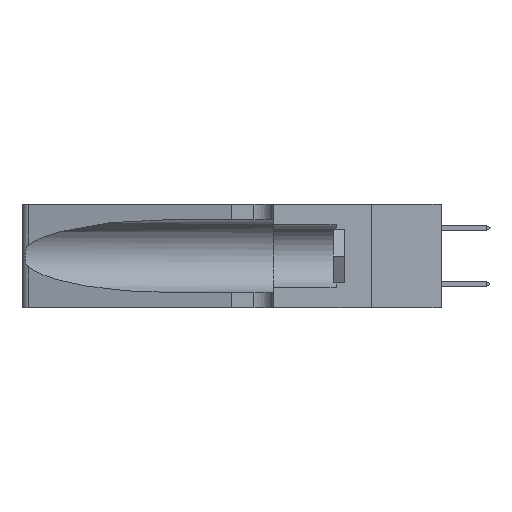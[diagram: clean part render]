
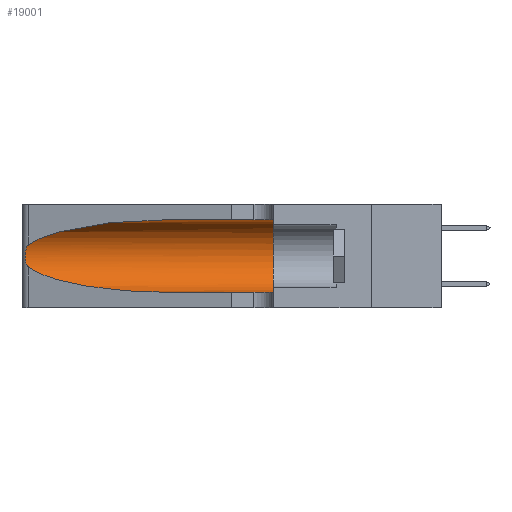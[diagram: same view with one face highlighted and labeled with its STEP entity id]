
A CAD part, left-side view. The second image highlights one B-rep face of the part: STEP entity #19001.
In plain terms, the highlighted cylindrical face has radius 3.308 mm (diameter 6.617 mm), a partial arc.
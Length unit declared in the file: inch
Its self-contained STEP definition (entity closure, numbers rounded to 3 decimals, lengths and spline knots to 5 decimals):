
#551 = ORIENTED_EDGE ( 'NONE', *, *, #17460, .T. ) ;
#641 = CARTESIAN_POINT ( 'NONE',  ( 0.25487, 1.22718, 0.14631 ) ) ;
#1133 =( BOUNDED_CURVE ( )  B_SPLINE_CURVE ( 3, ( #2060, #19327, #19222, #4439 ),
 .UNSPECIFIED., .F., .T. ) 
 B_SPLINE_CURVE_WITH_KNOTS ( ( 4, 4 ),
 ( 1.5708, 2.84003 ),
 .UNSPECIFIED. ) 
 CURVE ( )  GEOMETRIC_REPRESENTATION_ITEM ( )  RATIONAL_B_SPLINE_CURVE ( ( 1., 0.87, 0.87, 1. ) ) 
 REPRESENTATION_ITEM ( '' )  );
#1561 = CARTESIAN_POINT ( 'NONE',  ( 0.25555, 1.22993, 0.14849 ) ) ;
#1677 = CARTESIAN_POINT ( 'NONE',  ( 0.1305, 0.35, 0.185 ) ) ;
#1917 = EDGE_LOOP ( 'NONE', ( #7066, #551, #21271, #15717, #28326, #12097 ) ) ;
#2060 = CARTESIAN_POINT ( 'NONE',  ( 0.1305, 0.72297, 0.31525 ) ) ;
#2667 = EDGE_CURVE ( 'NONE', #29819, #5821, #16450, .T. ) ;
#3539 = FACE_OUTER_BOUND ( 'NONE', #1917, .T. ) ;
#4139 = VERTEX_POINT ( 'NONE', #7620 ) ;
#4439 = CARTESIAN_POINT ( 'NONE',  ( 0.25487, 1.22718, 0.22369 ) ) ;
#4511 = B_SPLINE_CURVE_WITH_KNOTS ( 'NONE', 3,
 ( #25887, #30851, #11072, #16334, #6303, #11182, #23590, #28400, #13532, #23703, #26225, #11397, #1561, #16020 ),
 .UNSPECIFIED., .F., .F.,
 ( 4, 2, 2, 2, 2, 2, 4 ),
 ( 0., 0.00027, 0.00053, 0.00107, 0.0016, 0.00187, 0.00214 ),
 .UNSPECIFIED. ) ;
#4860 = EDGE_CURVE ( 'NONE', #20494, #13696, #8228, .T. ) ;
#4925 = CARTESIAN_POINT ( 'NONE',  ( 0.1305, 0.35, 0.05475 ) ) ;
#5821 = VERTEX_POINT ( 'NONE', #4925 ) ;
#6303 = CARTESIAN_POINT ( 'NONE',  ( 0.25854, 1.2359, 0.20912 ) ) ;
#7066 = ORIENTED_EDGE ( 'NONE', *, *, #11610, .T. ) ;
#7512 = VERTEX_POINT ( 'NONE', #26462 ) ;
#7620 = CARTESIAN_POINT ( 'NONE',  ( 0.25487, 1.22718, 0.22369 ) ) ;
#8002 = CARTESIAN_POINT ( 'NONE',  ( 0.18966, 0.96281, 0.05475 ) ) ;
#8224 = DIRECTION ( 'NONE',  ( 0., -1., 0. ) ) ;
#8228 = LINE ( 'NONE', #12948, #19827 ) ;
#8367 = DIRECTION ( 'NONE',  ( 0., -1., 0. ) ) ;
#10428 = CARTESIAN_POINT ( 'NONE',  ( 0.1305, 1.61858, 0.05475 ) ) ;
#11072 = CARTESIAN_POINT ( 'NONE',  ( 0.25639, 1.23184, 0.21858 ) ) ;
#11182 = CARTESIAN_POINT ( 'NONE',  ( 0.26018, 1.23835, 0.19895 ) ) ;
#11397 = CARTESIAN_POINT ( 'NONE',  ( 0.25639, 1.23186, 0.15144 ) ) ;
#11610 = EDGE_CURVE ( 'NONE', #20494, #4139, #1133, .T. ) ;
#11839 = DIRECTION ( 'NONE',  ( 0., 0., -1. ) ) ;
#12097 = ORIENTED_EDGE ( 'NONE', *, *, #4860, .F. ) ;
#12313 = EDGE_CURVE ( 'NONE', #7512, #29819, #27517, .T. ) ;
#12948 = CARTESIAN_POINT ( 'NONE',  ( 0.1305, 1.61858, 0.31525 ) ) ;
#12983 = CIRCLE ( 'NONE', #24735, 0.13025 ) ;
#13532 = CARTESIAN_POINT ( 'NONE',  ( 0.26017, 1.23833, 0.17102 ) ) ;
#13696 = VERTEX_POINT ( 'NONE', #23753 ) ;
#15717 = ORIENTED_EDGE ( 'NONE', *, *, #2667, .T. ) ;
#16020 = CARTESIAN_POINT ( 'NONE',  ( 0.25487, 1.22718, 0.14631 ) ) ;
#16334 = CARTESIAN_POINT ( 'NONE',  ( 0.25787, 1.23484, 0.2124 ) ) ;
#16450 = LINE ( 'NONE', #10428, #30763 ) ;
#17032 = CARTESIAN_POINT ( 'NONE',  ( 0.1305, 0.72297, 0.05475 ) ) ;
#17460 = EDGE_CURVE ( 'NONE', #4139, #7512, #4511, .T. ) ;
#18965 = CARTESIAN_POINT ( 'NONE',  ( 0.1305, 1.61858, 0.185 ) ) ;
#19001 = ADVANCED_FACE ( 'NONE', ( #3539 ), #24434, .F. ) ;
#19050 = DIRECTION ( 'NONE',  ( 0., 0., 1. ) ) ;
#19222 = CARTESIAN_POINT ( 'NONE',  ( 0.2373, 1.15595, 0.28018 ) ) ;
#19327 = CARTESIAN_POINT ( 'NONE',  ( 0.18966, 0.96281, 0.31525 ) ) ;
#19827 = VECTOR ( 'NONE', #8224, 39.37008 ) ;
#20494 = VERTEX_POINT ( 'NONE', #23167 ) ;
#21271 = ORIENTED_EDGE ( 'NONE', *, *, #12313, .T. ) ;
#21365 = AXIS2_PLACEMENT_3D ( 'NONE', #18965, #26683, #11839 ) ;
#21381 = EDGE_CURVE ( 'NONE', #13696, #5821, #12983, .T. ) ;
#23167 = CARTESIAN_POINT ( 'NONE',  ( 0.1305, 0.72297, 0.31525 ) ) ;
#23590 = CARTESIAN_POINT ( 'NONE',  ( 0.26075, 1.23896, 0.19203 ) ) ;
#23703 = CARTESIAN_POINT ( 'NONE',  ( 0.25856, 1.23593, 0.16098 ) ) ;
#23753 = CARTESIAN_POINT ( 'NONE',  ( 0.1305, 0.35, 0.31525 ) ) ;
#23822 = DIRECTION ( 'NONE',  ( 0., 1., 0. ) ) ;
#24434 = CYLINDRICAL_SURFACE ( 'NONE', #21365, 0.13025 ) ;
#24735 = AXIS2_PLACEMENT_3D ( 'NONE', #1677, #23822, #19050 ) ;
#25887 = CARTESIAN_POINT ( 'NONE',  ( 0.25487, 1.22718, 0.22369 ) ) ;
#26225 = CARTESIAN_POINT ( 'NONE',  ( 0.25789, 1.23486, 0.15765 ) ) ;
#26462 = CARTESIAN_POINT ( 'NONE',  ( 0.25487, 1.22718, 0.14631 ) ) ;
#26683 = DIRECTION ( 'NONE',  ( 0., -1., 0. ) ) ;
#27517 =( BOUNDED_CURVE ( )  B_SPLINE_CURVE ( 3, ( #641, #30055, #8002, #27719 ),
 .UNSPECIFIED., .F., .T. ) 
 B_SPLINE_CURVE_WITH_KNOTS ( ( 4, 4 ),
 ( 3.44316, 4.71239 ),
 .UNSPECIFIED. ) 
 CURVE ( )  GEOMETRIC_REPRESENTATION_ITEM ( )  RATIONAL_B_SPLINE_CURVE ( ( 1., 0.87, 0.87, 1. ) ) 
 REPRESENTATION_ITEM ( '' )  );
#27719 = CARTESIAN_POINT ( 'NONE',  ( 0.1305, 0.72297, 0.05475 ) ) ;
#28326 = ORIENTED_EDGE ( 'NONE', *, *, #21381, .F. ) ;
#28400 = CARTESIAN_POINT ( 'NONE',  ( 0.26075, 1.23896, 0.178 ) ) ;
#29819 = VERTEX_POINT ( 'NONE', #17032 ) ;
#30055 = CARTESIAN_POINT ( 'NONE',  ( 0.2373, 1.15595, 0.08982 ) ) ;
#30763 = VECTOR ( 'NONE', #8367, 39.37008 ) ;
#30851 = CARTESIAN_POINT ( 'NONE',  ( 0.25555, 1.22994, 0.2215 ) ) ;
